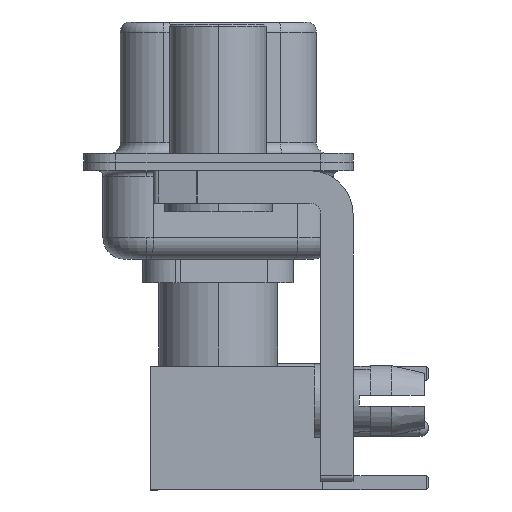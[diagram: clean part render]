
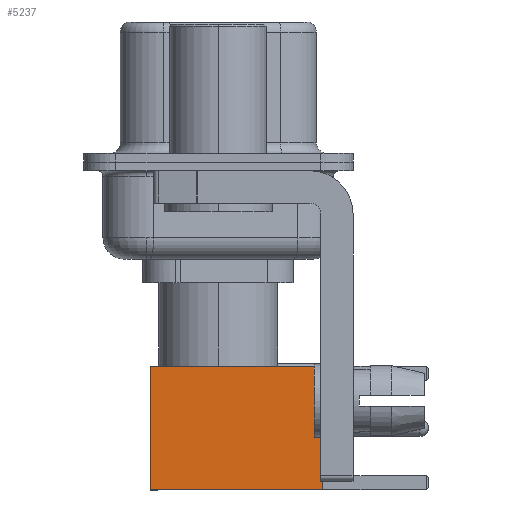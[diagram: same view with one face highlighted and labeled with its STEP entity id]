
A CAD part, left-side view. The second image highlights one B-rep face of the part: STEP entity #5237.
In plain terms, the highlighted face is planar.
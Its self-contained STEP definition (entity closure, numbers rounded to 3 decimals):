
#1243 = VECTOR ( 'NONE', #23592, 1000. ) ;
#1565 = EDGE_LOOP ( 'NONE', ( #17264, #15176, #10873, #16934 ) ) ;
#5237 = ADVANCED_FACE ( 'NONE', ( #29130 ), #17855, .T. ) ;
#5309 = CARTESIAN_POINT ( 'NONE',  ( -2.875, 2.875, 8. ) ) ;
#6414 = EDGE_CURVE ( 'NONE', #16671, #16758, #25813, .T. ) ;
#8151 = VERTEX_POINT ( 'NONE', #24353 ) ;
#10441 = CARTESIAN_POINT ( 'NONE',  ( 2.875, 2.875, 8. ) ) ;
#10873 = ORIENTED_EDGE ( 'NONE', *, *, #6414, .F. ) ;
#11175 = CARTESIAN_POINT ( 'NONE',  ( 2.875, 2.875, 0. ) ) ;
#12578 = DIRECTION ( 'NONE',  ( -1., 0., 0. ) ) ;
#13568 = LINE ( 'NONE', #11175, #21193 ) ;
#15176 = ORIENTED_EDGE ( 'NONE', *, *, #20219, .T. ) ;
#15383 = DIRECTION ( 'NONE',  ( 0., 0., -1. ) ) ;
#16212 = CARTESIAN_POINT ( 'NONE',  ( 0., 2.875, 0. ) ) ;
#16671 = VERTEX_POINT ( 'NONE', #5309 ) ;
#16758 = VERTEX_POINT ( 'NONE', #17349 ) ;
#16934 = ORIENTED_EDGE ( 'NONE', *, *, #19070, .F. ) ;
#17264 = ORIENTED_EDGE ( 'NONE', *, *, #17479, .T. ) ;
#17349 = CARTESIAN_POINT ( 'NONE',  ( -2.875, 2.875, 0. ) ) ;
#17479 = EDGE_CURVE ( 'NONE', #19620, #8151, #13568, .T. ) ;
#17855 = PLANE ( 'NONE',  #21298 ) ;
#19070 = EDGE_CURVE ( 'NONE', #19620, #16671, #21648, .T. ) ;
#19133 = CARTESIAN_POINT ( 'NONE',  ( 0., 2.875, 8. ) ) ;
#19620 = VERTEX_POINT ( 'NONE', #10441 ) ;
#20219 = EDGE_CURVE ( 'NONE', #8151, #16758, #21213, .T. ) ;
#21193 = VECTOR ( 'NONE', #15383, 1000. ) ;
#21213 = LINE ( 'NONE', #16212, #24352 ) ;
#21298 = AXIS2_PLACEMENT_3D ( 'NONE', #26895, #21872, #23931 ) ;
#21648 = LINE ( 'NONE', #19133, #29254 ) ;
#21872 = DIRECTION ( 'NONE',  ( 0., 1., 0. ) ) ;
#23015 = CARTESIAN_POINT ( 'NONE',  ( -2.875, 2.875, 0. ) ) ;
#23592 = DIRECTION ( 'NONE',  ( 0., 0., -1. ) ) ;
#23931 = DIRECTION ( 'NONE',  ( 0., 0., 1. ) ) ;
#24352 = VECTOR ( 'NONE', #12578, 1000. ) ;
#24353 = CARTESIAN_POINT ( 'NONE',  ( 2.875, 2.875, 0. ) ) ;
#25644 = DIRECTION ( 'NONE',  ( -1., 0., 0. ) ) ;
#25813 = LINE ( 'NONE', #23015, #1243 ) ;
#26895 = CARTESIAN_POINT ( 'NONE',  ( 2.875, 2.875, 0. ) ) ;
#29130 = FACE_OUTER_BOUND ( 'NONE', #1565, .T. ) ;
#29254 = VECTOR ( 'NONE', #25644, 1000. ) ;
